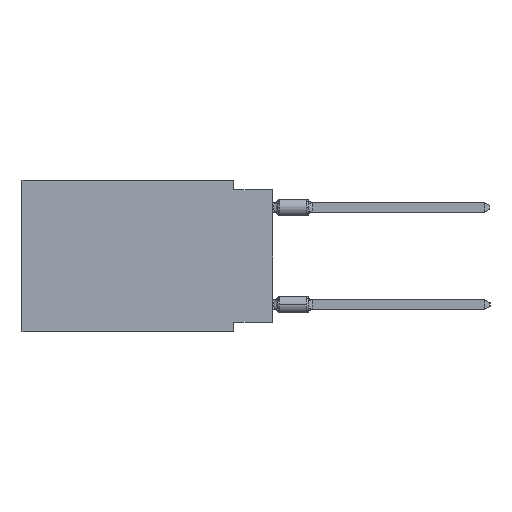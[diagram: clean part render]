
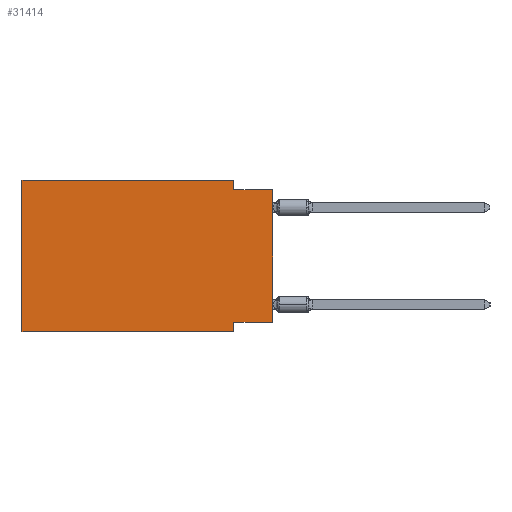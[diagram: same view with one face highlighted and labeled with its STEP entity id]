
A CAD part, left-side view. The second image highlights one B-rep face of the part: STEP entity #31414.
In plain terms, the highlighted planar face has unit normal (-1, 0, 0).
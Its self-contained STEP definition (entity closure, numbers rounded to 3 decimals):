
#137 = VECTOR ( 'NONE', #13371, 1000. ) ;
#1330 = CARTESIAN_POINT ( 'NONE',  ( 0., 2.54, -9.906 ) ) ;
#1606 = VECTOR ( 'NONE', #9416, 1000. ) ;
#1757 = CARTESIAN_POINT ( 'NONE',  ( 0., 2.54, 0. ) ) ;
#2450 = CARTESIAN_POINT ( 'NONE',  ( 0., 2.54, -9.271 ) ) ;
#2906 = VERTEX_POINT ( 'NONE', #24145 ) ;
#3624 = CARTESIAN_POINT ( 'NONE',  ( 0., 16.383, 0. ) ) ;
#4654 = EDGE_CURVE ( 'NONE', #2906, #33886, #28048, .T. ) ;
#4739 = EDGE_CURVE ( 'NONE', #14658, #2906, #22819, .T. ) ;
#5571 = PLANE ( 'NONE',  #24283 ) ;
#6951 = LINE ( 'NONE', #24163, #25534 ) ;
#7156 = VECTOR ( 'NONE', #21770, 1000. ) ;
#9303 = VERTEX_POINT ( 'NONE', #30538 ) ;
#9416 = DIRECTION ( 'NONE',  ( 0., 0., 1. ) ) ;
#10244 = ORIENTED_EDGE ( 'NONE', *, *, #10898, .F. ) ;
#10411 = EDGE_CURVE ( 'NONE', #27059, #10657, #20133, .T. ) ;
#10657 = VERTEX_POINT ( 'NONE', #1330 ) ;
#10898 = EDGE_CURVE ( 'NONE', #9303, #31618, #24103, .T. ) ;
#11739 = ORIENTED_EDGE ( 'NONE', *, *, #17702, .F. ) ;
#13371 = DIRECTION ( 'NONE',  ( 0., -1., 0. ) ) ;
#14087 = FACE_OUTER_BOUND ( 'NONE', #26148, .T. ) ;
#14658 = VERTEX_POINT ( 'NONE', #19441 ) ;
#14896 = DIRECTION ( 'NONE',  ( 0., -1., 0. ) ) ;
#15059 = DIRECTION ( 'NONE',  ( 0., 0., 1. ) ) ;
#15534 = ORIENTED_EDGE ( 'NONE', *, *, #29090, .T. ) ;
#16020 = EDGE_CURVE ( 'NONE', #20342, #33886, #29943, .T. ) ;
#16054 = CARTESIAN_POINT ( 'NONE',  ( 0., 0., -0.635 ) ) ;
#16459 = ORIENTED_EDGE ( 'NONE', *, *, #18279, .F. ) ;
#16993 = DIRECTION ( 'NONE',  ( 1., 0., 0. ) ) ;
#17702 = EDGE_CURVE ( 'NONE', #31618, #14658, #6951, .T. ) ;
#18279 = EDGE_CURVE ( 'NONE', #20342, #27059, #30381, .T. ) ;
#19441 = CARTESIAN_POINT ( 'NONE',  ( 0., 2.54, 0. ) ) ;
#20133 = LINE ( 'NONE', #37695, #22203 ) ;
#20342 = VERTEX_POINT ( 'NONE', #33951 ) ;
#20651 = DIRECTION ( 'NONE',  ( 0., 0., -1. ) ) ;
#21008 = CARTESIAN_POINT ( 'NONE',  ( 0., 0., -0.635 ) ) ;
#21589 = LINE ( 'NONE', #24864, #7156 ) ;
#21770 = DIRECTION ( 'NONE',  ( 0., -1., 0. ) ) ;
#22085 = CARTESIAN_POINT ( 'NONE',  ( 0., 0., -9.271 ) ) ;
#22203 = VECTOR ( 'NONE', #23015, 1000. ) ;
#22286 = ORIENTED_EDGE ( 'NONE', *, *, #16020, .T. ) ;
#22819 = LINE ( 'NONE', #1757, #28520 ) ;
#23015 = DIRECTION ( 'NONE',  ( 0., 0., -1. ) ) ;
#24103 = LINE ( 'NONE', #3624, #1606 ) ;
#24145 = CARTESIAN_POINT ( 'NONE',  ( 0., 2.54, -0.635 ) ) ;
#24163 = CARTESIAN_POINT ( 'NONE',  ( 0., 16.383, 0. ) ) ;
#24283 = AXIS2_PLACEMENT_3D ( 'NONE', #35140, #16993, #20651 ) ;
#24864 = CARTESIAN_POINT ( 'NONE',  ( 0., 16.383, -9.906 ) ) ;
#25437 = ORIENTED_EDGE ( 'NONE', *, *, #10411, .F. ) ;
#25534 = VECTOR ( 'NONE', #14896, 1000. ) ;
#26148 = EDGE_LOOP ( 'NONE', ( #22286, #30266, #34859, #11739, #10244, #15534, #25437, #16459 ) ) ;
#26815 = VECTOR ( 'NONE', #28266, 1000. ) ;
#27059 = VERTEX_POINT ( 'NONE', #2450 ) ;
#28048 = LINE ( 'NONE', #16054, #137 ) ;
#28266 = DIRECTION ( 'NONE',  ( 0., 1., 0. ) ) ;
#28520 = VECTOR ( 'NONE', #31319, 1000. ) ;
#29090 = EDGE_CURVE ( 'NONE', #9303, #10657, #21589, .T. ) ;
#29739 = CARTESIAN_POINT ( 'NONE',  ( 0., 0., 0. ) ) ;
#29943 = LINE ( 'NONE', #29739, #34724 ) ;
#30266 = ORIENTED_EDGE ( 'NONE', *, *, #4654, .F. ) ;
#30381 = LINE ( 'NONE', #22085, #26815 ) ;
#30538 = CARTESIAN_POINT ( 'NONE',  ( 0., 16.383, -9.906 ) ) ;
#31319 = DIRECTION ( 'NONE',  ( 0., 0., -1. ) ) ;
#31414 = ADVANCED_FACE ( 'NONE', ( #14087 ), #5571, .F. ) ;
#31498 = CARTESIAN_POINT ( 'NONE',  ( 0., 16.383, 0. ) ) ;
#31618 = VERTEX_POINT ( 'NONE', #31498 ) ;
#33886 = VERTEX_POINT ( 'NONE', #21008 ) ;
#33951 = CARTESIAN_POINT ( 'NONE',  ( 0., 0., -9.271 ) ) ;
#34724 = VECTOR ( 'NONE', #15059, 1000. ) ;
#34859 = ORIENTED_EDGE ( 'NONE', *, *, #4739, .F. ) ;
#35140 = CARTESIAN_POINT ( 'NONE',  ( 0., 16.383, 0. ) ) ;
#37695 = CARTESIAN_POINT ( 'NONE',  ( 0., 2.54, -9.906 ) ) ;
